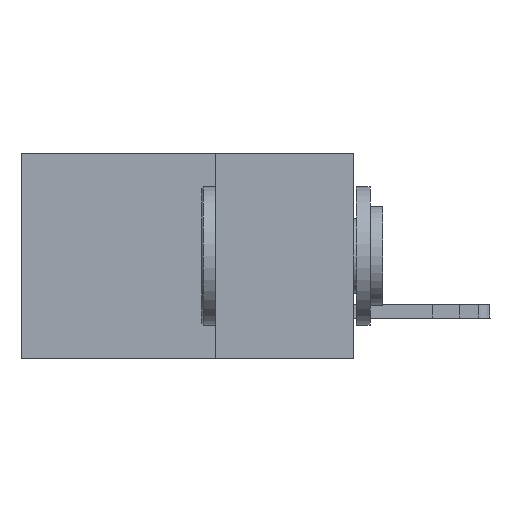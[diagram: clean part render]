
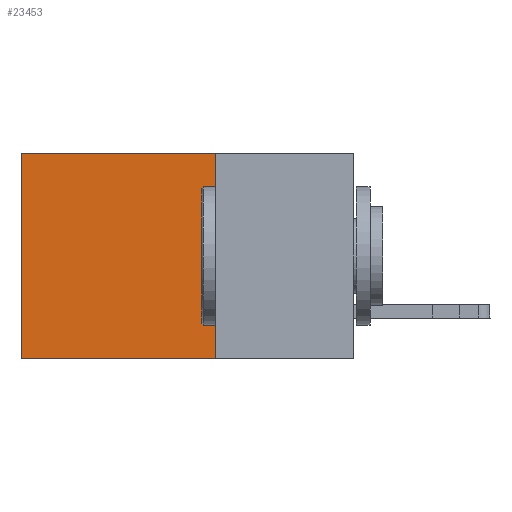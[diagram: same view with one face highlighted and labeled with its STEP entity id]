
A CAD part, left-side view. The second image highlights one B-rep face of the part: STEP entity #23453.
In plain terms, the highlighted planar face has unit normal (-1, 0, 0).
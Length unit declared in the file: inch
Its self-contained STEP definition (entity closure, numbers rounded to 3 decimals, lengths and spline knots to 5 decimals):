
#1004 = EDGE_CURVE ( 'NONE', #29951, #11409, #12098, .T. ) ;
#1048 = ORIENTED_EDGE ( 'NONE', *, *, #35069, .T. ) ;
#1563 = LINE ( 'NONE', #11334, #30205 ) ;
#3610 = CARTESIAN_POINT ( 'NONE',  ( 0.2875, 0.6, -0.37 ) ) ;
#6519 = CARTESIAN_POINT ( 'NONE',  ( 0.2875, 0.25, 0. ) ) ;
#6522 = DIRECTION ( 'NONE',  ( 0., 0., -1. ) ) ;
#6638 = DIRECTION ( 'NONE',  ( 0., 1., 0. ) ) ;
#7142 = VERTEX_POINT ( 'NONE', #35381 ) ;
#7532 = VECTOR ( 'NONE', #6638, 39.37008 ) ;
#9350 = VERTEX_POINT ( 'NONE', #34842 ) ;
#10585 = FACE_OUTER_BOUND ( 'NONE', #14797, .T. ) ;
#10608 = CARTESIAN_POINT ( 'NONE',  ( 0.2875, 0.25, 0. ) ) ;
#11334 = CARTESIAN_POINT ( 'NONE',  ( 0.2875, 0.25, 0. ) ) ;
#11409 = VERTEX_POINT ( 'NONE', #3610 ) ;
#12098 = LINE ( 'NONE', #21095, #18693 ) ;
#14138 = DIRECTION ( 'NONE',  ( 0., 0., -1. ) ) ;
#14797 = EDGE_LOOP ( 'NONE', ( #34622, #31257, #17832, #1048 ) ) ;
#14923 = VECTOR ( 'NONE', #6522, 39.37008 ) ;
#14930 = LINE ( 'NONE', #6519, #7532 ) ;
#16198 = DIRECTION ( 'NONE',  ( 0., 0., -1. ) ) ;
#17832 = ORIENTED_EDGE ( 'NONE', *, *, #17943, .F. ) ;
#17943 = EDGE_CURVE ( 'NONE', #7142, #29951, #1563, .T. ) ;
#18693 = VECTOR ( 'NONE', #29429, 39.37008 ) ;
#21095 = CARTESIAN_POINT ( 'NONE',  ( 0.2875, 0.25, -0.37 ) ) ;
#21182 = AXIS2_PLACEMENT_3D ( 'NONE', #10608, #32817, #16198 ) ;
#21495 = LINE ( 'NONE', #25998, #14923 ) ;
#23453 = ADVANCED_FACE ( 'NONE', ( #10585 ), #30025, .F. ) ;
#25998 = CARTESIAN_POINT ( 'NONE',  ( 0.2875, 0.6, 0. ) ) ;
#26090 = EDGE_CURVE ( 'NONE', #9350, #11409, #21495, .T. ) ;
#29429 = DIRECTION ( 'NONE',  ( 0., 1., 0. ) ) ;
#29951 = VERTEX_POINT ( 'NONE', #32956 ) ;
#30025 = PLANE ( 'NONE',  #21182 ) ;
#30205 = VECTOR ( 'NONE', #14138, 39.37008 ) ;
#31257 = ORIENTED_EDGE ( 'NONE', *, *, #1004, .F. ) ;
#32817 = DIRECTION ( 'NONE',  ( 1., 0., 0. ) ) ;
#32956 = CARTESIAN_POINT ( 'NONE',  ( 0.2875, 0.25, -0.37 ) ) ;
#34622 = ORIENTED_EDGE ( 'NONE', *, *, #26090, .T. ) ;
#34842 = CARTESIAN_POINT ( 'NONE',  ( 0.2875, 0.6, 0. ) ) ;
#35069 = EDGE_CURVE ( 'NONE', #7142, #9350, #14930, .T. ) ;
#35381 = CARTESIAN_POINT ( 'NONE',  ( 0.2875, 0.25, 0. ) ) ;
